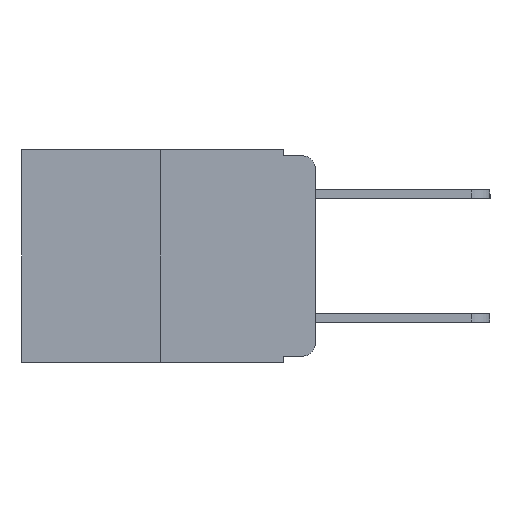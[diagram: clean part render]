
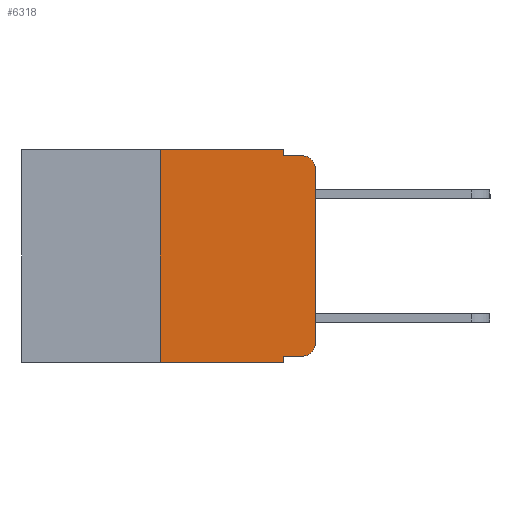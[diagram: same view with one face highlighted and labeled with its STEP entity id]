
A CAD part, left-side view. The second image highlights one B-rep face of the part: STEP entity #6318.
In plain terms, the highlighted planar face has unit normal (-1, 0, 0).
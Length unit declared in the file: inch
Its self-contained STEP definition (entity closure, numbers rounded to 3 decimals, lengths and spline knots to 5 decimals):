
#209 = ORIENTED_EDGE ( 'NONE', *, *, #17943, .T. ) ;
#623 = VERTEX_POINT ( 'NONE', #16518 ) ;
#720 = FACE_OUTER_BOUND ( 'NONE', #19618, .T. ) ;
#1237 = CARTESIAN_POINT ( 'NONE',  ( 0., 0.02, -0.313 ) ) ;
#1268 = ORIENTED_EDGE ( 'NONE', *, *, #17834, .F. ) ;
#1761 = PLANE ( 'NONE',  #1796 ) ;
#1795 = CIRCLE ( 'NONE', #15966, 0.02 ) ;
#1796 = AXIS2_PLACEMENT_3D ( 'NONE', #3162, #15610, #20725 ) ;
#1848 = DIRECTION ( 'NONE',  ( 0., -1., 0. ) ) ;
#2037 = VECTOR ( 'NONE', #8337, 39.37008 ) ;
#2525 = EDGE_CURVE ( 'NONE', #15042, #10409, #1795, .T. ) ;
#2672 = VECTOR ( 'NONE', #1848, 39.37008 ) ;
#2695 = VERTEX_POINT ( 'NONE', #19950 ) ;
#3040 = DIRECTION ( 'NONE',  ( 0., 0., -1. ) ) ;
#3074 = VERTEX_POINT ( 'NONE', #14929 ) ;
#3162 = CARTESIAN_POINT ( 'NONE',  ( 0., 0.473, 0. ) ) ;
#3328 = ORIENTED_EDGE ( 'NONE', *, *, #9810, .T. ) ;
#3669 = VERTEX_POINT ( 'NONE', #13930 ) ;
#4349 = LINE ( 'NONE', #7775, #16456 ) ;
#4659 = VERTEX_POINT ( 'NONE', #10908 ) ;
#4955 = DIRECTION ( 'NONE',  ( 0., -1., 0. ) ) ;
#5028 = CARTESIAN_POINT ( 'NONE',  ( 0., 0.25, 0. ) ) ;
#5396 = ORIENTED_EDGE ( 'NONE', *, *, #9213, .T. ) ;
#5498 = CARTESIAN_POINT ( 'NONE',  ( 0., 0.051, 0. ) ) ;
#6318 = ADVANCED_FACE ( 'NONE', ( #720 ), #1761, .F. ) ;
#6584 = CARTESIAN_POINT ( 'NONE',  ( 0., 0.051, -0.333 ) ) ;
#6797 = VECTOR ( 'NONE', #18417, 39.37008 ) ;
#7109 = ORIENTED_EDGE ( 'NONE', *, *, #11841, .F. ) ;
#7140 = DIRECTION ( 'NONE',  ( 0., 0., -1. ) ) ;
#7209 = VECTOR ( 'NONE', #20279, 39.37008 ) ;
#7555 = DIRECTION ( 'NONE',  ( 0., 0., 1. ) ) ;
#7775 = CARTESIAN_POINT ( 'NONE',  ( 0., 0.051, 0. ) ) ;
#7843 = DIRECTION ( 'NONE',  ( 0., 0., -1. ) ) ;
#7870 = CARTESIAN_POINT ( 'NONE',  ( 0., 0.051, -0.01 ) ) ;
#8337 = DIRECTION ( 'NONE',  ( 0., 0., 1. ) ) ;
#8620 = CARTESIAN_POINT ( 'NONE',  ( 0., 0., 0. ) ) ;
#8788 = CARTESIAN_POINT ( 'NONE',  ( 0., 0.02, -0.03 ) ) ;
#8920 = ORIENTED_EDGE ( 'NONE', *, *, #14152, .F. ) ;
#9213 = EDGE_CURVE ( 'NONE', #11228, #3074, #19291, .T. ) ;
#9810 = EDGE_CURVE ( 'NONE', #4659, #15042, #18291, .T. ) ;
#9862 = VECTOR ( 'NONE', #4955, 39.37008 ) ;
#9940 = CARTESIAN_POINT ( 'NONE',  ( 0., 0.473, 0. ) ) ;
#10013 = ORIENTED_EDGE ( 'NONE', *, *, #17437, .F. ) ;
#10409 = VERTEX_POINT ( 'NONE', #10935 ) ;
#10695 = ORIENTED_EDGE ( 'NONE', *, *, #16064, .F. ) ;
#10908 = CARTESIAN_POINT ( 'NONE',  ( 0., 0., -0.313 ) ) ;
#10935 = CARTESIAN_POINT ( 'NONE',  ( 0., 0.02, -0.01 ) ) ;
#11228 = VERTEX_POINT ( 'NONE', #6584 ) ;
#11411 = ORIENTED_EDGE ( 'NONE', *, *, #17855, .T. ) ;
#11461 = DIRECTION ( 'NONE',  ( 0., 0., -1. ) ) ;
#11841 = EDGE_CURVE ( 'NONE', #14692, #10409, #20128, .T. ) ;
#12057 = ORIENTED_EDGE ( 'NONE', *, *, #2525, .T. ) ;
#12406 = LINE ( 'NONE', #5498, #20262 ) ;
#12501 = DIRECTION ( 'NONE',  ( -1., 0., 0. ) ) ;
#13127 = VERTEX_POINT ( 'NONE', #16128 ) ;
#13930 = CARTESIAN_POINT ( 'NONE',  ( 0., 0.25, -0.343 ) ) ;
#14061 = CARTESIAN_POINT ( 'NONE',  ( 0., 0., -0.03 ) ) ;
#14111 = VECTOR ( 'NONE', #7555, 39.37008 ) ;
#14152 = EDGE_CURVE ( 'NONE', #11228, #623, #12406, .T. ) ;
#14448 = CARTESIAN_POINT ( 'NONE',  ( 0., 0.051, -0.333 ) ) ;
#14692 = VERTEX_POINT ( 'NONE', #17742 ) ;
#14762 = LINE ( 'NONE', #5028, #2037 ) ;
#14929 = CARTESIAN_POINT ( 'NONE',  ( 0., 0.02, -0.333 ) ) ;
#15042 = VERTEX_POINT ( 'NONE', #14061 ) ;
#15339 = LINE ( 'NONE', #9940, #2672 ) ;
#15610 = DIRECTION ( 'NONE',  ( 1., 0., 0. ) ) ;
#15966 = AXIS2_PLACEMENT_3D ( 'NONE', #8788, #19665, #11461 ) ;
#15976 = CIRCLE ( 'NONE', #16668, 0.02 ) ;
#16006 = CARTESIAN_POINT ( 'NONE',  ( 0., 0.473, -0.343 ) ) ;
#16064 = EDGE_CURVE ( 'NONE', #2695, #13127, #15339, .T. ) ;
#16128 = CARTESIAN_POINT ( 'NONE',  ( 0., 0.051, 0. ) ) ;
#16456 = VECTOR ( 'NONE', #7843, 39.37008 ) ;
#16518 = CARTESIAN_POINT ( 'NONE',  ( 0., 0.051, -0.343 ) ) ;
#16668 = AXIS2_PLACEMENT_3D ( 'NONE', #1237, #12501, #3040 ) ;
#17437 = EDGE_CURVE ( 'NONE', #3669, #2695, #14762, .T. ) ;
#17742 = CARTESIAN_POINT ( 'NONE',  ( 0., 0.051, -0.01 ) ) ;
#17834 = EDGE_CURVE ( 'NONE', #13127, #14692, #4349, .T. ) ;
#17855 = EDGE_CURVE ( 'NONE', #3074, #4659, #15976, .T. ) ;
#17943 = EDGE_CURVE ( 'NONE', #3669, #623, #18165, .T. ) ;
#18165 = LINE ( 'NONE', #16006, #9862 ) ;
#18291 = LINE ( 'NONE', #8620, #14111 ) ;
#18417 = DIRECTION ( 'NONE',  ( 0., -1., 0. ) ) ;
#19291 = LINE ( 'NONE', #14448, #6797 ) ;
#19618 = EDGE_LOOP ( 'NONE', ( #3328, #12057, #7109, #1268, #10695, #10013, #209, #8920, #5396, #11411 ) ) ;
#19665 = DIRECTION ( 'NONE',  ( -1., 0., 0. ) ) ;
#19950 = CARTESIAN_POINT ( 'NONE',  ( 0., 0.25, 0. ) ) ;
#20128 = LINE ( 'NONE', #7870, #7209 ) ;
#20262 = VECTOR ( 'NONE', #7140, 39.37008 ) ;
#20279 = DIRECTION ( 'NONE',  ( 0., -1., 0. ) ) ;
#20725 = DIRECTION ( 'NONE',  ( 0., 0., -1. ) ) ;
